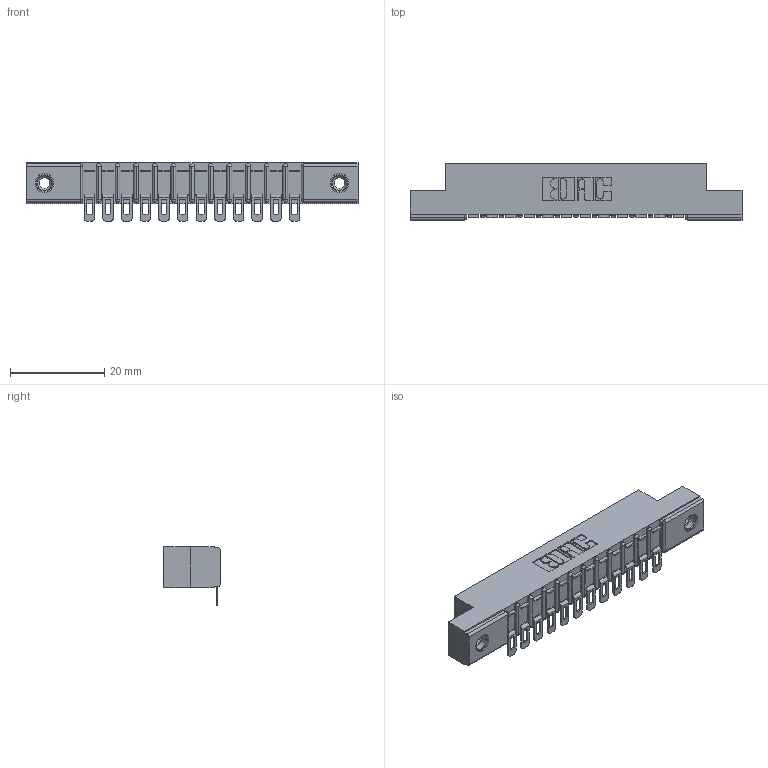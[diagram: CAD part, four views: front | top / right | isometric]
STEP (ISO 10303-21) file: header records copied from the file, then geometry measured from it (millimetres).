
FILE_DESCRIPTION (( 'STEP AP203' ), '1' );
FILE_NAME ('307-012-554-108.STEP', '2019-09-04T19:58:14', ( '' ), ( '' ), 'SwSTEP 2.0', 'SolidWorks 2016', '' );
FILE_SCHEMA (( 'CONFIG_CONTROL_DESIGN' ));
Length unit declared in the file: inch
Products named in the file (4): 307 Part_.156 Dia Mounting Holes; 307-012-554-108; 345-250-001_345-250-003-102; 307-290-002_554
Assembly tree (15 placements, depth 2):
  307-012-554-108
    307 Part_.156 Dia Mounting Holes
    307-290-002_554  x12
    345-250-001_345-250-003-102  x2
Bounding box: 70.56 x 12.01 x 12.52 mm (x, y, z)
Volume: 4650.9 mm3; surface area: 7971.2 mm2
Topology: 15 solids, 15 shells, 1163 faces, 3495 edges, 2286 vertices
Faces by surface type: plane 654, cylinder 467, sphere 26, cone 12, torus 4
Entity records: 16136 total; most frequent: CARTESIAN_POINT 2697, ORIENTED_EDGE 2680, DIRECTION 2650, EDGE_CURVE 1340, LINE 1004, VECTOR 1004, VERTEX_POINT 870, AXIS2_PLACEMENT_3D 823
